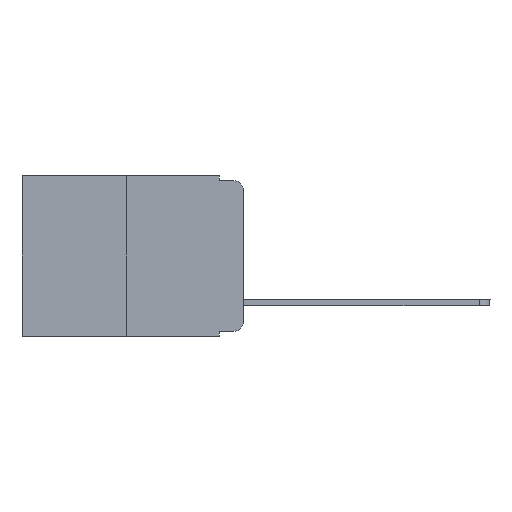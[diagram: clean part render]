
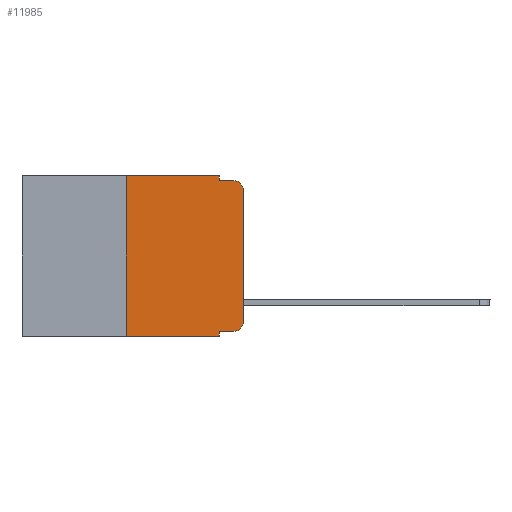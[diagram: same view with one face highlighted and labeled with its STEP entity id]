
A CAD part, left-side view. The second image highlights one B-rep face of the part: STEP entity #11985.
In plain terms, the highlighted planar face has unit normal (-1, 0, 0).
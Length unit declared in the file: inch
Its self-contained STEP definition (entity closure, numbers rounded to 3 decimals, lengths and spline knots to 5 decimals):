
#208 = CARTESIAN_POINT ( 'NONE',  ( 0., 0., -0.313 ) ) ;
#250 = DIRECTION ( 'NONE',  ( 0., -1., 0. ) ) ;
#319 = DIRECTION ( 'NONE',  ( 0., -1., 0. ) ) ;
#407 = LINE ( 'NONE', #7465, #3898 ) ;
#553 = ORIENTED_EDGE ( 'NONE', *, *, #10980, .F. ) ;
#799 = VERTEX_POINT ( 'NONE', #208 ) ;
#881 = CARTESIAN_POINT ( 'NONE',  ( 0., 0.25, 0. ) ) ;
#898 = VERTEX_POINT ( 'NONE', #15639 ) ;
#1008 = VECTOR ( 'NONE', #11117, 39.37008 ) ;
#1372 = CARTESIAN_POINT ( 'NONE',  ( 0., 0.473, 0. ) ) ;
#1612 = VECTOR ( 'NONE', #18029, 39.37008 ) ;
#2048 = EDGE_LOOP ( 'NONE', ( #6298, #15739, #9127, #553, #4919, #10942, #11091, #9086, #13617, #14416 ) ) ;
#2251 = CARTESIAN_POINT ( 'NONE',  ( 0., 0., 0. ) ) ;
#2551 = VERTEX_POINT ( 'NONE', #4121 ) ;
#3024 = EDGE_CURVE ( 'NONE', #17010, #14420, #14232, .T. ) ;
#3263 = EDGE_CURVE ( 'NONE', #898, #16059, #16253, .T. ) ;
#3338 = CARTESIAN_POINT ( 'NONE',  ( 0., 0.02, -0.313 ) ) ;
#3502 = VERTEX_POINT ( 'NONE', #6244 ) ;
#3513 = DIRECTION ( 'NONE',  ( 0., 0., -1. ) ) ;
#3745 = DIRECTION ( 'NONE',  ( 0., -1., 0. ) ) ;
#3898 = VECTOR ( 'NONE', #6079, 39.37008 ) ;
#3933 = FACE_OUTER_BOUND ( 'NONE', #2048, .T. ) ;
#4121 = CARTESIAN_POINT ( 'NONE',  ( 0., 0.051, 0. ) ) ;
#4754 = EDGE_CURVE ( 'NONE', #8788, #2551, #6093, .T. ) ;
#4814 = CARTESIAN_POINT ( 'NONE',  ( 0., 0.051, -0.333 ) ) ;
#4919 = ORIENTED_EDGE ( 'NONE', *, *, #4754, .F. ) ;
#5261 = CARTESIAN_POINT ( 'NONE',  ( 0., 0.051, -0.343 ) ) ;
#5416 = CARTESIAN_POINT ( 'NONE',  ( 0., 0.051, 0. ) ) ;
#5537 = CARTESIAN_POINT ( 'NONE',  ( 0., 0.25, 0. ) ) ;
#5564 = DIRECTION ( 'NONE',  ( 1., 0., 0. ) ) ;
#5892 = LINE ( 'NONE', #11470, #7441 ) ;
#6079 = DIRECTION ( 'NONE',  ( 0., 0., -1. ) ) ;
#6093 = LINE ( 'NONE', #15865, #15379 ) ;
#6162 = CARTESIAN_POINT ( 'NONE',  ( 0., 0.02, -0.333 ) ) ;
#6166 = EDGE_CURVE ( 'NONE', #799, #3502, #14859, .T. ) ;
#6244 = CARTESIAN_POINT ( 'NONE',  ( 0., 0., -0.03 ) ) ;
#6298 = ORIENTED_EDGE ( 'NONE', *, *, #6166, .T. ) ;
#6814 = CARTESIAN_POINT ( 'NONE',  ( 0., 0.02, -0.01 ) ) ;
#7441 = VECTOR ( 'NONE', #14305, 39.37008 ) ;
#7465 = CARTESIAN_POINT ( 'NONE',  ( 0., 0.051, 0. ) ) ;
#7729 = DIRECTION ( 'NONE',  ( -1., 0., 0. ) ) ;
#8788 = VERTEX_POINT ( 'NONE', #881 ) ;
#8842 = EDGE_CURVE ( 'NONE', #3502, #16059, #11751, .T. ) ;
#9086 = ORIENTED_EDGE ( 'NONE', *, *, #9169, .F. ) ;
#9127 = ORIENTED_EDGE ( 'NONE', *, *, #3263, .F. ) ;
#9169 = EDGE_CURVE ( 'NONE', #17010, #17165, #407, .T. ) ;
#9246 = EDGE_CURVE ( 'NONE', #14420, #799, #14684, .T. ) ;
#9609 = CARTESIAN_POINT ( 'NONE',  ( 0., 0.25, -0.343 ) ) ;
#9730 = AXIS2_PLACEMENT_3D ( 'NONE', #3338, #7729, #3513 ) ;
#10013 = AXIS2_PLACEMENT_3D ( 'NONE', #15972, #10763, #14674 ) ;
#10325 = EDGE_CURVE ( 'NONE', #15023, #8788, #16691, .T. ) ;
#10481 = EDGE_CURVE ( 'NONE', #15023, #17165, #5892, .T. ) ;
#10763 = DIRECTION ( 'NONE',  ( -1., 0., 0. ) ) ;
#10942 = ORIENTED_EDGE ( 'NONE', *, *, #10325, .F. ) ;
#10980 = EDGE_CURVE ( 'NONE', #2551, #898, #16468, .T. ) ;
#11091 = ORIENTED_EDGE ( 'NONE', *, *, #10481, .T. ) ;
#11117 = DIRECTION ( 'NONE',  ( 0., 0., 1. ) ) ;
#11470 = CARTESIAN_POINT ( 'NONE',  ( 0., 0.473, -0.343 ) ) ;
#11751 = CIRCLE ( 'NONE', #10013, 0.02 ) ;
#11985 = ADVANCED_FACE ( 'NONE', ( #3933 ), #17818, .F. ) ;
#12440 = DIRECTION ( 'NONE',  ( 0., 0., -1. ) ) ;
#12857 = CARTESIAN_POINT ( 'NONE',  ( 0., 0.051, -0.333 ) ) ;
#13294 = VECTOR ( 'NONE', #3745, 39.37008 ) ;
#13617 = ORIENTED_EDGE ( 'NONE', *, *, #3024, .T. ) ;
#14062 = VECTOR ( 'NONE', #16137, 39.37008 ) ;
#14232 = LINE ( 'NONE', #12857, #15915 ) ;
#14305 = DIRECTION ( 'NONE',  ( 0., -1., 0. ) ) ;
#14416 = ORIENTED_EDGE ( 'NONE', *, *, #9246, .T. ) ;
#14420 = VERTEX_POINT ( 'NONE', #6162 ) ;
#14674 = DIRECTION ( 'NONE',  ( 0., 0., -1. ) ) ;
#14684 = CIRCLE ( 'NONE', #9730, 0.02 ) ;
#14859 = LINE ( 'NONE', #2251, #14062 ) ;
#14971 = AXIS2_PLACEMENT_3D ( 'NONE', #1372, #5564, #12440 ) ;
#15023 = VERTEX_POINT ( 'NONE', #9609 ) ;
#15379 = VECTOR ( 'NONE', #250, 39.37008 ) ;
#15639 = CARTESIAN_POINT ( 'NONE',  ( 0., 0.051, -0.01 ) ) ;
#15739 = ORIENTED_EDGE ( 'NONE', *, *, #8842, .T. ) ;
#15865 = CARTESIAN_POINT ( 'NONE',  ( 0., 0.473, 0. ) ) ;
#15915 = VECTOR ( 'NONE', #319, 39.37008 ) ;
#15972 = CARTESIAN_POINT ( 'NONE',  ( 0., 0.02, -0.03 ) ) ;
#16059 = VERTEX_POINT ( 'NONE', #6814 ) ;
#16137 = DIRECTION ( 'NONE',  ( 0., 0., 1. ) ) ;
#16253 = LINE ( 'NONE', #17442, #13294 ) ;
#16468 = LINE ( 'NONE', #5416, #1612 ) ;
#16691 = LINE ( 'NONE', #5537, #1008 ) ;
#17010 = VERTEX_POINT ( 'NONE', #4814 ) ;
#17165 = VERTEX_POINT ( 'NONE', #5261 ) ;
#17442 = CARTESIAN_POINT ( 'NONE',  ( 0., 0.051, -0.01 ) ) ;
#17818 = PLANE ( 'NONE',  #14971 ) ;
#18029 = DIRECTION ( 'NONE',  ( 0., 0., -1. ) ) ;
